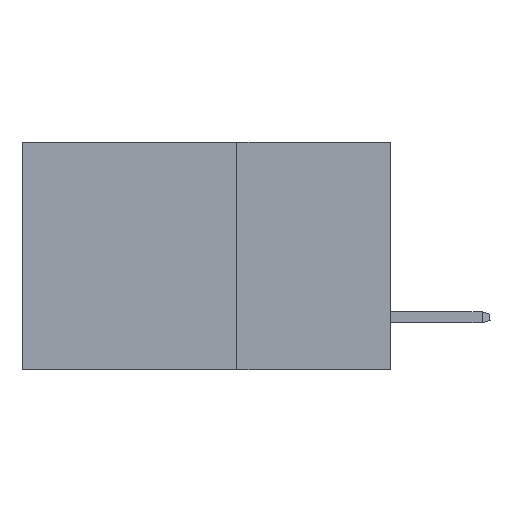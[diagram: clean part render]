
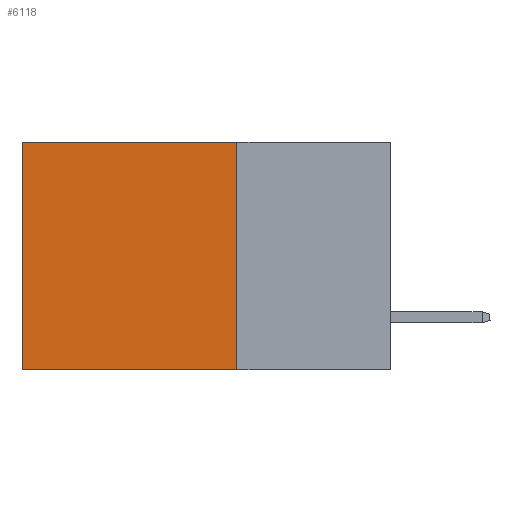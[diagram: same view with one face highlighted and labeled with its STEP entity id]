
A CAD part, left-side view. The second image highlights one B-rep face of the part: STEP entity #6118.
In plain terms, the highlighted planar face has unit normal (-1, 0, 0).
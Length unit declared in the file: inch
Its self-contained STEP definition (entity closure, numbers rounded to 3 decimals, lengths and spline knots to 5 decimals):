
#244 = LINE ( 'NONE', #1485, #4930 ) ;
#493 = DIRECTION ( 'NONE',  ( 0., 1., 0. ) ) ;
#964 = VERTEX_POINT ( 'NONE', #4306 ) ;
#982 = DIRECTION ( 'NONE',  ( 1., 0., 0. ) ) ;
#990 = EDGE_CURVE ( 'NONE', #12344, #2980, #1160, .T. ) ;
#1160 = LINE ( 'NONE', #3332, #3129 ) ;
#1485 = CARTESIAN_POINT ( 'NONE',  ( 0.2875, 0.25, 0. ) ) ;
#1736 = VERTEX_POINT ( 'NONE', #6687 ) ;
#1996 = ORIENTED_EDGE ( 'NONE', *, *, #990, .T. ) ;
#2399 = CARTESIAN_POINT ( 'NONE',  ( 0.2875, 0.25, 0. ) ) ;
#2575 = DIRECTION ( 'NONE',  ( 0., 0., -1. ) ) ;
#2618 = CARTESIAN_POINT ( 'NONE',  ( 0.2875, 0.25, -0.37 ) ) ;
#2926 = DIRECTION ( 'NONE',  ( 0., 0., -1. ) ) ;
#2980 = VERTEX_POINT ( 'NONE', #12021 ) ;
#3129 = VECTOR ( 'NONE', #3376, 39.37008 ) ;
#3132 = EDGE_CURVE ( 'NONE', #964, #12344, #12168, .T. ) ;
#3332 = CARTESIAN_POINT ( 'NONE',  ( 0.2875, 0.6, 0. ) ) ;
#3376 = DIRECTION ( 'NONE',  ( 0., 0., -1. ) ) ;
#3611 = CARTESIAN_POINT ( 'NONE',  ( 0.2875, 0.6, 0. ) ) ;
#4108 = VECTOR ( 'NONE', #11400, 39.37008 ) ;
#4250 = ORIENTED_EDGE ( 'NONE', *, *, #8030, .F. ) ;
#4306 = CARTESIAN_POINT ( 'NONE',  ( 0.2875, 0.25, 0. ) ) ;
#4458 = EDGE_LOOP ( 'NONE', ( #1996, #4250, #5504, #10005 ) ) ;
#4878 = LINE ( 'NONE', #2618, #4108 ) ;
#4930 = VECTOR ( 'NONE', #2575, 39.37008 ) ;
#5504 = ORIENTED_EDGE ( 'NONE', *, *, #11564, .F. ) ;
#5765 = PLANE ( 'NONE',  #7307 ) ;
#5804 = CARTESIAN_POINT ( 'NONE',  ( 0.2875, 0.25, 0. ) ) ;
#6118 = ADVANCED_FACE ( 'NONE', ( #7584 ), #5765, .F. ) ;
#6687 = CARTESIAN_POINT ( 'NONE',  ( 0.2875, 0.25, -0.37 ) ) ;
#7141 = VECTOR ( 'NONE', #493, 39.37008 ) ;
#7307 = AXIS2_PLACEMENT_3D ( 'NONE', #5804, #982, #2926 ) ;
#7584 = FACE_OUTER_BOUND ( 'NONE', #4458, .T. ) ;
#8030 = EDGE_CURVE ( 'NONE', #1736, #2980, #4878, .T. ) ;
#10005 = ORIENTED_EDGE ( 'NONE', *, *, #3132, .T. ) ;
#11400 = DIRECTION ( 'NONE',  ( 0., 1., 0. ) ) ;
#11564 = EDGE_CURVE ( 'NONE', #964, #1736, #244, .T. ) ;
#12021 = CARTESIAN_POINT ( 'NONE',  ( 0.2875, 0.6, -0.37 ) ) ;
#12168 = LINE ( 'NONE', #2399, #7141 ) ;
#12344 = VERTEX_POINT ( 'NONE', #3611 ) ;
